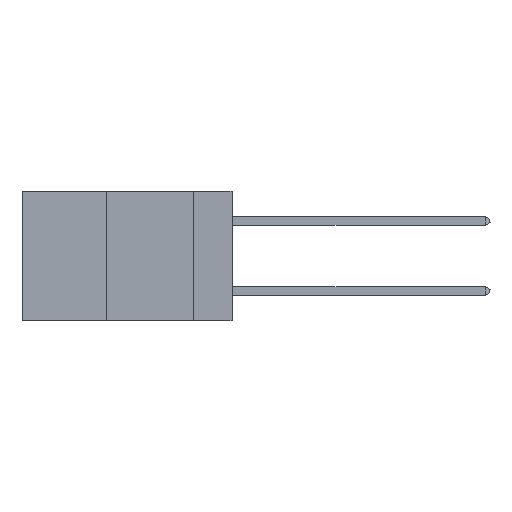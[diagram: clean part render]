
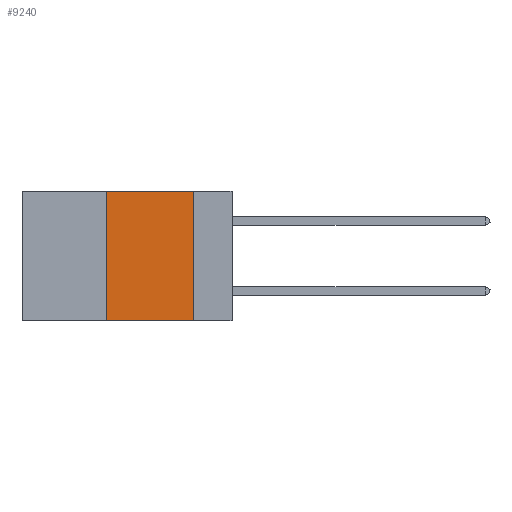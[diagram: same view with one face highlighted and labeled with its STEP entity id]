
A CAD part, left-side view. The second image highlights one B-rep face of the part: STEP entity #9240.
In plain terms, the highlighted planar face has unit normal (-1, 0, 0).
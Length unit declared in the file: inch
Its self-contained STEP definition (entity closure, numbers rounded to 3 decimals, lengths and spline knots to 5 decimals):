
#472 = VERTEX_POINT ( 'NONE', #1627 ) ;
#642 = DIRECTION ( 'NONE',  ( 0., 0., 1. ) ) ;
#1627 = CARTESIAN_POINT ( 'NONE',  ( 0., 0.11, -0.37 ) ) ;
#1716 = CARTESIAN_POINT ( 'NONE',  ( 0., 0.11, 0. ) ) ;
#3344 = VERTEX_POINT ( 'NONE', #23549 ) ;
#4531 = ORIENTED_EDGE ( 'NONE', *, *, #20986, .F. ) ;
#5739 = PLANE ( 'NONE',  #9212 ) ;
#5831 = DIRECTION ( 'NONE',  ( 0., 0., -1. ) ) ;
#7048 = FACE_OUTER_BOUND ( 'NONE', #23794, .T. ) ;
#7164 = LINE ( 'NONE', #24971, #22623 ) ;
#7172 = VECTOR ( 'NONE', #26132, 39.37008 ) ;
#8052 = CARTESIAN_POINT ( 'NONE',  ( 0., 0.6, -0.37 ) ) ;
#8101 = LINE ( 'NONE', #1716, #13525 ) ;
#8883 = DIRECTION ( 'NONE',  ( 0., -1., 0. ) ) ;
#8892 = EDGE_CURVE ( 'NONE', #3344, #21831, #20636, .T. ) ;
#9212 = AXIS2_PLACEMENT_3D ( 'NONE', #15938, #17974, #5831 ) ;
#9240 = ADVANCED_FACE ( 'NONE', ( #7048 ), #5739, .F. ) ;
#10334 = CARTESIAN_POINT ( 'NONE',  ( 0., 0.36, -0.37 ) ) ;
#12419 = EDGE_CURVE ( 'NONE', #19729, #472, #12598, .T. ) ;
#12598 = LINE ( 'NONE', #8052, #7172 ) ;
#13118 = ORIENTED_EDGE ( 'NONE', *, *, #12419, .T. ) ;
#13525 = VECTOR ( 'NONE', #23955, 39.37008 ) ;
#14900 = CARTESIAN_POINT ( 'NONE',  ( 0., 0.6, 0. ) ) ;
#15938 = CARTESIAN_POINT ( 'NONE',  ( 0., 0.6, 0. ) ) ;
#16481 = EDGE_CURVE ( 'NONE', #19729, #3344, #7164, .T. ) ;
#16975 = CARTESIAN_POINT ( 'NONE',  ( 0., 0.11, 0. ) ) ;
#17974 = DIRECTION ( 'NONE',  ( 1., 0., 0. ) ) ;
#19685 = ORIENTED_EDGE ( 'NONE', *, *, #8892, .F. ) ;
#19729 = VERTEX_POINT ( 'NONE', #10334 ) ;
#20015 = VECTOR ( 'NONE', #8883, 39.37008 ) ;
#20636 = LINE ( 'NONE', #14900, #20015 ) ;
#20986 = EDGE_CURVE ( 'NONE', #21831, #472, #8101, .T. ) ;
#21831 = VERTEX_POINT ( 'NONE', #16975 ) ;
#22623 = VECTOR ( 'NONE', #642, 39.37008 ) ;
#22735 = ORIENTED_EDGE ( 'NONE', *, *, #16481, .F. ) ;
#23549 = CARTESIAN_POINT ( 'NONE',  ( 0., 0.36, 0. ) ) ;
#23794 = EDGE_LOOP ( 'NONE', ( #4531, #19685, #22735, #13118 ) ) ;
#23955 = DIRECTION ( 'NONE',  ( 0., 0., -1. ) ) ;
#24971 = CARTESIAN_POINT ( 'NONE',  ( 0., 0.36, 0. ) ) ;
#26132 = DIRECTION ( 'NONE',  ( 0., -1., 0. ) ) ;
